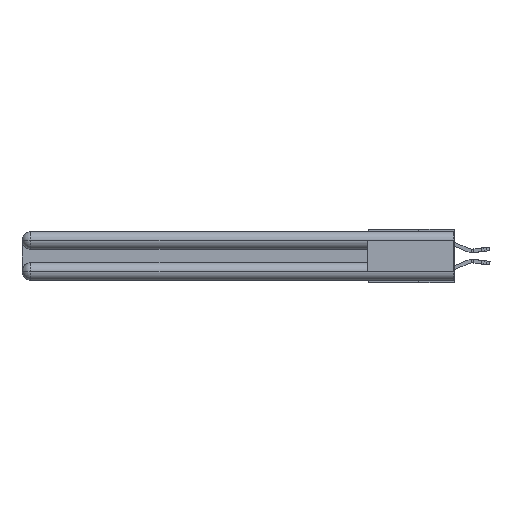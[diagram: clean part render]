
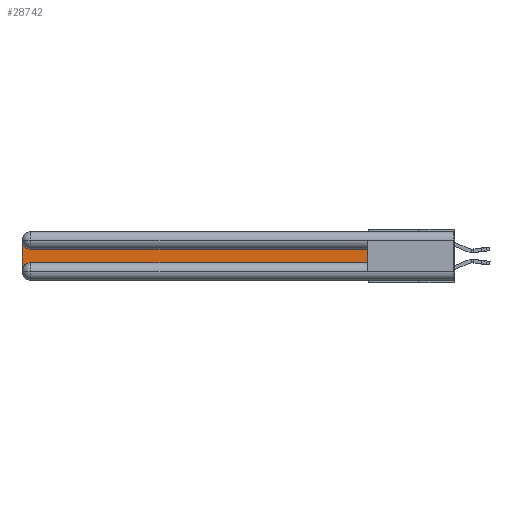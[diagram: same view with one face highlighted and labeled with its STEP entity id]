
A CAD part, left-side view. The second image highlights one B-rep face of the part: STEP entity #28742.
In plain terms, the highlighted planar face has unit normal (-1, 0, 0).
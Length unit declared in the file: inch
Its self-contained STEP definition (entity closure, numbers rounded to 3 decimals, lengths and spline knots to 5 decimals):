
#241 = EDGE_CURVE ( 'NONE', #23165, #2867, #1723, .T. ) ;
#332 = ORIENTED_EDGE ( 'NONE', *, *, #241, .T. ) ;
#1485 = ORIENTED_EDGE ( 'NONE', *, *, #8077, .T. ) ;
#1723 = LINE ( 'NONE', #9213, #29277 ) ;
#1790 = AXIS2_PLACEMENT_3D ( 'NONE', #27960, #8857, #13756 ) ;
#1871 = CARTESIAN_POINT ( 'NONE',  ( 0.075, 3., -0.0625 ) ) ;
#2867 = VERTEX_POINT ( 'NONE', #6631 ) ;
#3516 = AXIS2_PLACEMENT_3D ( 'NONE', #27362, #3659, #15615 ) ;
#3659 = DIRECTION ( 'NONE',  ( 1., 0., 0. ) ) ;
#4111 = EDGE_CURVE ( 'NONE', #13920, #22560, #4871, .T. ) ;
#4871 = CIRCLE ( 'NONE', #3516, 0.06 ) ;
#5533 = CARTESIAN_POINT ( 'NONE',  ( 0.075, 3., -0.1225 ) ) ;
#6569 = DIRECTION ( 'NONE',  ( 0., 0., 1. ) ) ;
#6587 = LINE ( 'NONE', #27274, #9503 ) ;
#6631 = CARTESIAN_POINT ( 'NONE',  ( 0.075, 0.6, -0.2175 ) ) ;
#7067 = VECTOR ( 'NONE', #11711, 39.37008 ) ;
#8077 = EDGE_CURVE ( 'NONE', #30080, #23165, #11935, .T. ) ;
#8840 = VECTOR ( 'NONE', #21875, 39.37008 ) ;
#8857 = DIRECTION ( 'NONE',  ( 1., 0., 0. ) ) ;
#9213 = CARTESIAN_POINT ( 'NONE',  ( 0.075, 0.6, -0.2175 ) ) ;
#9503 = VECTOR ( 'NONE', #6569, 39.37008 ) ;
#9880 = VERTEX_POINT ( 'NONE', #25770 ) ;
#10140 = EDGE_CURVE ( 'NONE', #9880, #13920, #23877, .T. ) ;
#11143 = CARTESIAN_POINT ( 'NONE',  ( 0.075, 0.6, -0.1225 ) ) ;
#11711 = DIRECTION ( 'NONE',  ( 0., 0., -1. ) ) ;
#11935 = CIRCLE ( 'NONE', #1790, 0.06 ) ;
#13272 = LINE ( 'NONE', #25526, #7067 ) ;
#13756 = DIRECTION ( 'NONE',  ( 0., 0., -1. ) ) ;
#13920 = VERTEX_POINT ( 'NONE', #15103 ) ;
#14704 = PLANE ( 'NONE',  #19741 ) ;
#15103 = CARTESIAN_POINT ( 'NONE',  ( 0.075, 2.94, -0.1225 ) ) ;
#15615 = DIRECTION ( 'NONE',  ( 0., 0., -1. ) ) ;
#17267 = DIRECTION ( 'NONE',  ( 1., 0., 0. ) ) ;
#17983 = EDGE_LOOP ( 'NONE', ( #26991, #29916, #28949, #1485, #332, #18891 ) ) ;
#18891 = ORIENTED_EDGE ( 'NONE', *, *, #20225, .T. ) ;
#19741 = AXIS2_PLACEMENT_3D ( 'NONE', #5533, #17267, #26742 ) ;
#20225 = EDGE_CURVE ( 'NONE', #2867, #9880, #6587, .T. ) ;
#20828 = DIRECTION ( 'NONE',  ( 0., -1., 0. ) ) ;
#21875 = DIRECTION ( 'NONE',  ( 0., 1., 0. ) ) ;
#22560 = VERTEX_POINT ( 'NONE', #1871 ) ;
#23165 = VERTEX_POINT ( 'NONE', #25647 ) ;
#23877 = LINE ( 'NONE', #11143, #8840 ) ;
#24810 = EDGE_CURVE ( 'NONE', #22560, #30080, #13272, .T. ) ;
#25020 = FACE_OUTER_BOUND ( 'NONE', #17983, .T. ) ;
#25526 = CARTESIAN_POINT ( 'NONE',  ( 0.075, 3., -0.2175 ) ) ;
#25647 = CARTESIAN_POINT ( 'NONE',  ( 0.075, 2.94, -0.2175 ) ) ;
#25770 = CARTESIAN_POINT ( 'NONE',  ( 0.075, 0.6, -0.1225 ) ) ;
#26742 = DIRECTION ( 'NONE',  ( 0., 0., -1. ) ) ;
#26991 = ORIENTED_EDGE ( 'NONE', *, *, #10140, .T. ) ;
#27274 = CARTESIAN_POINT ( 'NONE',  ( 0.075, 0.6, -0.2175 ) ) ;
#27362 = CARTESIAN_POINT ( 'NONE',  ( 0.075, 2.94, -0.0625 ) ) ;
#27960 = CARTESIAN_POINT ( 'NONE',  ( 0.075, 2.94, -0.2775 ) ) ;
#28637 = CARTESIAN_POINT ( 'NONE',  ( 0.075, 3., -0.2775 ) ) ;
#28742 = ADVANCED_FACE ( 'NONE', ( #25020 ), #14704, .F. ) ;
#28949 = ORIENTED_EDGE ( 'NONE', *, *, #24810, .T. ) ;
#29277 = VECTOR ( 'NONE', #20828, 39.37008 ) ;
#29916 = ORIENTED_EDGE ( 'NONE', *, *, #4111, .T. ) ;
#30080 = VERTEX_POINT ( 'NONE', #28637 ) ;
